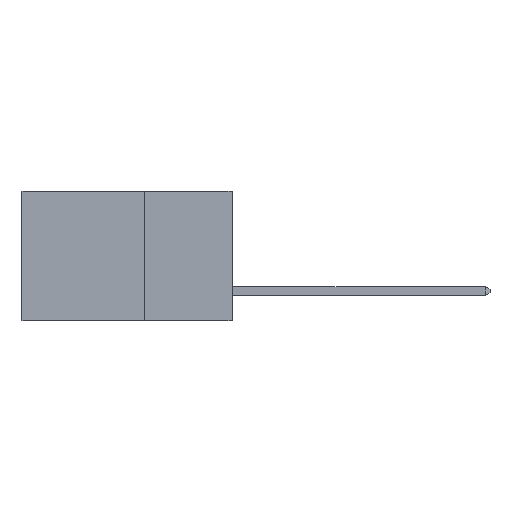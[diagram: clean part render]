
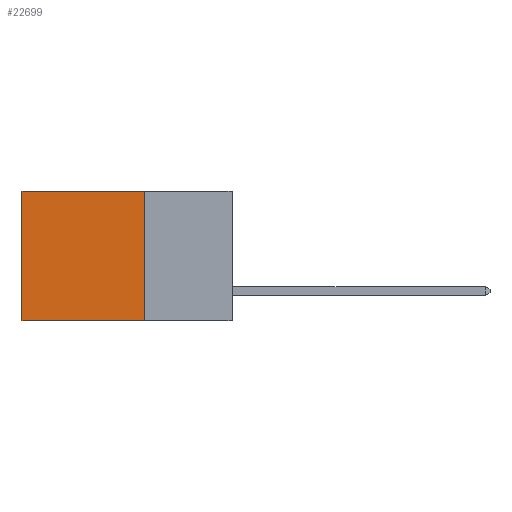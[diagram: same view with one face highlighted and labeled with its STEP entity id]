
A CAD part, left-side view. The second image highlights one B-rep face of the part: STEP entity #22699.
In plain terms, the highlighted planar face has unit normal (-1, 0, 0).
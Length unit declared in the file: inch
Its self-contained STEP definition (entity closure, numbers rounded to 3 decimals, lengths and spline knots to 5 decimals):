
#348 = CARTESIAN_POINT ( 'NONE',  ( 0.2875, 0.25, 0. ) ) ;
#494 = CARTESIAN_POINT ( 'NONE',  ( 0.2875, 0.25, 0. ) ) ;
#635 = LINE ( 'NONE', #3392, #21717 ) ;
#933 = CARTESIAN_POINT ( 'NONE',  ( 0.2875, 0.25, 0. ) ) ;
#968 = CARTESIAN_POINT ( 'NONE',  ( 0.2875, 0.25, -0.37 ) ) ;
#1489 = ORIENTED_EDGE ( 'NONE', *, *, #3237, .F. ) ;
#2437 = DIRECTION ( 'NONE',  ( 0., 1., 0. ) ) ;
#3237 = EDGE_CURVE ( 'NONE', #11385, #18416, #17963, .T. ) ;
#3392 = CARTESIAN_POINT ( 'NONE',  ( 0.2875, 0.6, 0. ) ) ;
#3897 = ORIENTED_EDGE ( 'NONE', *, *, #19535, .T. ) ;
#4000 = EDGE_LOOP ( 'NONE', ( #24784, #5930, #1489, #3897 ) ) ;
#4729 = LINE ( 'NONE', #348, #20310 ) ;
#4851 = CARTESIAN_POINT ( 'NONE',  ( 0.2875, 0.25, 0. ) ) ;
#5930 = ORIENTED_EDGE ( 'NONE', *, *, #8442, .F. ) ;
#7218 = DIRECTION ( 'NONE',  ( 0., 0., -1. ) ) ;
#8442 = EDGE_CURVE ( 'NONE', #18416, #24620, #17227, .T. ) ;
#9344 = DIRECTION ( 'NONE',  ( 0., 1., 0. ) ) ;
#11385 = VERTEX_POINT ( 'NONE', #494 ) ;
#11737 = DIRECTION ( 'NONE',  ( 0., 0., -1. ) ) ;
#11934 = VERTEX_POINT ( 'NONE', #16465 ) ;
#11975 = VECTOR ( 'NONE', #9344, 39.37008 ) ;
#13308 = VECTOR ( 'NONE', #20573, 39.37008 ) ;
#16465 = CARTESIAN_POINT ( 'NONE',  ( 0.2875, 0.6, 0. ) ) ;
#16900 = AXIS2_PLACEMENT_3D ( 'NONE', #933, #19321, #7218 ) ;
#17227 = LINE ( 'NONE', #968, #11975 ) ;
#17268 = PLANE ( 'NONE',  #16900 ) ;
#17963 = LINE ( 'NONE', #4851, #13308 ) ;
#18415 = EDGE_CURVE ( 'NONE', #11934, #24620, #635, .T. ) ;
#18416 = VERTEX_POINT ( 'NONE', #23792 ) ;
#19321 = DIRECTION ( 'NONE',  ( 1., 0., 0. ) ) ;
#19535 = EDGE_CURVE ( 'NONE', #11385, #11934, #4729, .T. ) ;
#20071 = CARTESIAN_POINT ( 'NONE',  ( 0.2875, 0.6, -0.37 ) ) ;
#20310 = VECTOR ( 'NONE', #2437, 39.37008 ) ;
#20573 = DIRECTION ( 'NONE',  ( 0., 0., -1. ) ) ;
#20813 = FACE_OUTER_BOUND ( 'NONE', #4000, .T. ) ;
#21717 = VECTOR ( 'NONE', #11737, 39.37008 ) ;
#22699 = ADVANCED_FACE ( 'NONE', ( #20813 ), #17268, .F. ) ;
#23792 = CARTESIAN_POINT ( 'NONE',  ( 0.2875, 0.25, -0.37 ) ) ;
#24620 = VERTEX_POINT ( 'NONE', #20071 ) ;
#24784 = ORIENTED_EDGE ( 'NONE', *, *, #18415, .T. ) ;
